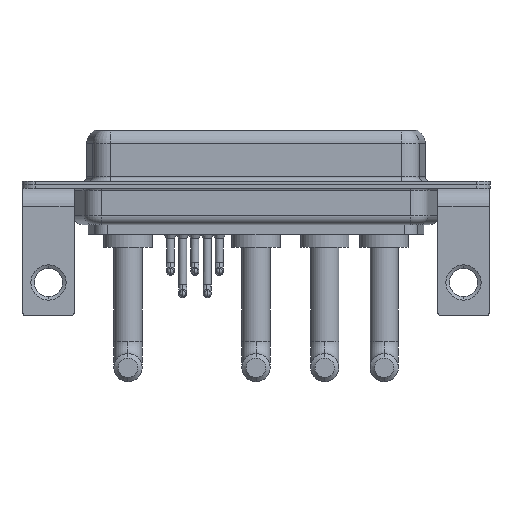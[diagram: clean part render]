
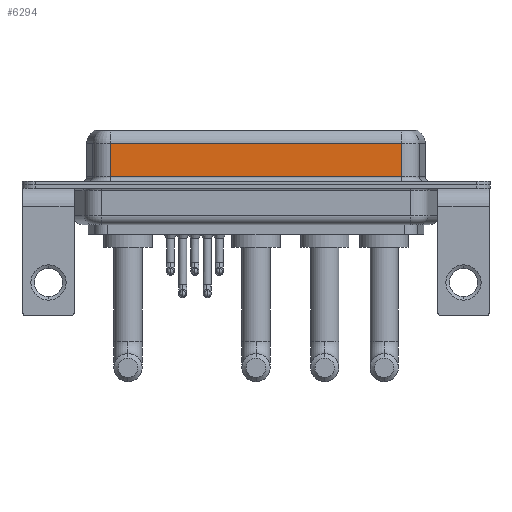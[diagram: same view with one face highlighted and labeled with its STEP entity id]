
A CAD part, front view. The second image highlights one B-rep face of the part: STEP entity #6294.
In plain terms, the highlighted planar face has unit normal (0, -1, 0).
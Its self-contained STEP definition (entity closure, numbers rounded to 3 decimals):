
#135 = VERTEX_POINT ( 'NONE', #5897 ) ;
#1209 = VECTOR ( 'NONE', #4114, 1000. ) ;
#1267 = AXIS2_PLACEMENT_3D ( 'NONE', #7409, #7110, #5631 ) ;
#1446 = PLANE ( 'NONE',  #1267 ) ;
#2589 = LINE ( 'NONE', #13718, #9659 ) ;
#2886 = ORIENTED_EDGE ( 'NONE', *, *, #14703, .F. ) ;
#3004 = CARTESIAN_POINT ( 'NONE',  ( 40.037, -3.95, 0.9 ) ) ;
#3272 = ORIENTED_EDGE ( 'NONE', *, *, #5354, .T. ) ;
#3400 = DIRECTION ( 'NONE',  ( 1., 0., 0. ) ) ;
#4114 = DIRECTION ( 'NONE',  ( 0., 0., -1. ) ) ;
#5354 = EDGE_CURVE ( 'NONE', #7536, #12545, #2589, .T. ) ;
#5631 = DIRECTION ( 'NONE',  ( 0., 0., 1. ) ) ;
#5897 = CARTESIAN_POINT ( 'NONE',  ( 7.013, -3.95, 0.9 ) ) ;
#6294 = ADVANCED_FACE ( 'NONE', ( #16857 ), #1446, .F. ) ;
#6521 = CARTESIAN_POINT ( 'NONE',  ( 40.037, -3.95, 4.65 ) ) ;
#7110 = DIRECTION ( 'NONE',  ( 0., 1., 0. ) ) ;
#7409 = CARTESIAN_POINT ( 'NONE',  ( 40.037, -3.95, 6.4 ) ) ;
#7536 = VERTEX_POINT ( 'NONE', #6521 ) ;
#8065 = LINE ( 'NONE', #17719, #1209 ) ;
#8728 = VERTEX_POINT ( 'NONE', #3004 ) ;
#9659 = VECTOR ( 'NONE', #11675, 1000. ) ;
#11103 = EDGE_CURVE ( 'NONE', #135, #8728, #15366, .T. ) ;
#11675 = DIRECTION ( 'NONE',  ( -1., 0., 0. ) ) ;
#12545 = VERTEX_POINT ( 'NONE', #17402 ) ;
#12618 = CARTESIAN_POINT ( 'NONE',  ( 40.037, -3.95, 0.9 ) ) ;
#12694 = VECTOR ( 'NONE', #3400, 1000. ) ;
#13718 = CARTESIAN_POINT ( 'NONE',  ( 40.037, -3.95, 4.65 ) ) ;
#13725 = ORIENTED_EDGE ( 'NONE', *, *, #18029, .T. ) ;
#13929 = DIRECTION ( 'NONE',  ( 0., 0., -1. ) ) ;
#14703 = EDGE_CURVE ( 'NONE', #7536, #8728, #16671, .T. ) ;
#15366 = LINE ( 'NONE', #12618, #12694 ) ;
#15392 = CARTESIAN_POINT ( 'NONE',  ( 40.037, -3.95, 6.4 ) ) ;
#15831 = EDGE_LOOP ( 'NONE', ( #2886, #3272, #13725, #17136 ) ) ;
#16671 = LINE ( 'NONE', #15392, #17194 ) ;
#16857 = FACE_OUTER_BOUND ( 'NONE', #15831, .T. ) ;
#17136 = ORIENTED_EDGE ( 'NONE', *, *, #11103, .T. ) ;
#17194 = VECTOR ( 'NONE', #13929, 1000. ) ;
#17402 = CARTESIAN_POINT ( 'NONE',  ( 7.013, -3.95, 4.65 ) ) ;
#17719 = CARTESIAN_POINT ( 'NONE',  ( 7.013, -3.95, 6.4 ) ) ;
#18029 = EDGE_CURVE ( 'NONE', #12545, #135, #8065, .T. ) ;
